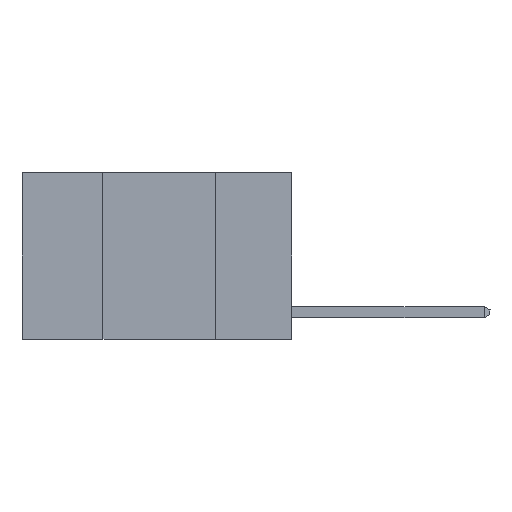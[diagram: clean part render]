
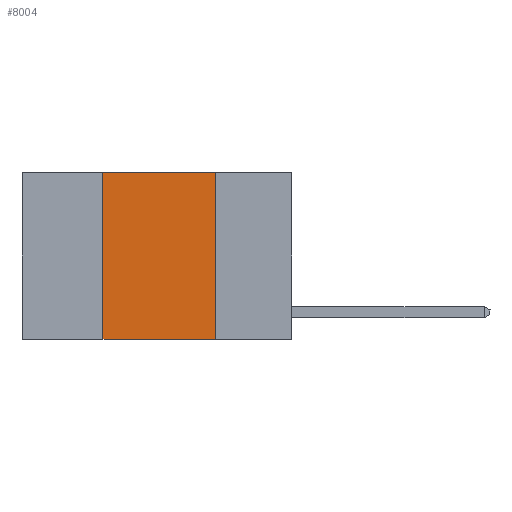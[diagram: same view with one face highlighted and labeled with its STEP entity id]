
A CAD part, left-side view. The second image highlights one B-rep face of the part: STEP entity #8004.
In plain terms, the highlighted planar face has unit normal (-1, 0, 0).
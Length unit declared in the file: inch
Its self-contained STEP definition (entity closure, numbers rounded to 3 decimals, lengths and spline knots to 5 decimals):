
#1813 = VERTEX_POINT ( 'NONE', #27494 ) ;
#3294 = LINE ( 'NONE', #10747, #24729 ) ;
#3376 = AXIS2_PLACEMENT_3D ( 'NONE', #18849, #20961, #8152 ) ;
#3519 = CARTESIAN_POINT ( 'NONE',  ( 0., 0.6, 0. ) ) ;
#3807 = ORIENTED_EDGE ( 'NONE', *, *, #9992, .F. ) ;
#5625 = EDGE_CURVE ( 'NONE', #9618, #1813, #24249, .T. ) ;
#6098 = VECTOR ( 'NONE', #22784, 39.37008 ) ;
#7294 = CARTESIAN_POINT ( 'NONE',  ( 0., 0.17, 0. ) ) ;
#7658 = CARTESIAN_POINT ( 'NONE',  ( 0., 0.42, 0. ) ) ;
#8004 = ADVANCED_FACE ( 'NONE', ( #25153 ), #18753, .F. ) ;
#8152 = DIRECTION ( 'NONE',  ( 0., 0., -1. ) ) ;
#8537 = EDGE_CURVE ( 'NONE', #16854, #9618, #11808, .T. ) ;
#9618 = VERTEX_POINT ( 'NONE', #18137 ) ;
#9623 = EDGE_LOOP ( 'NONE', ( #19580, #25844, #3807, #15947 ) ) ;
#9992 = EDGE_CURVE ( 'NONE', #15444, #16854, #3294, .T. ) ;
#10747 = CARTESIAN_POINT ( 'NONE',  ( 0., 0.42, 0. ) ) ;
#11808 = LINE ( 'NONE', #3519, #6098 ) ;
#12515 = CARTESIAN_POINT ( 'NONE',  ( 0., 0.42, -0.37 ) ) ;
#15436 = DIRECTION ( 'NONE',  ( 0., -1., 0. ) ) ;
#15444 = VERTEX_POINT ( 'NONE', #12515 ) ;
#15947 = ORIENTED_EDGE ( 'NONE', *, *, #21604, .T. ) ;
#16854 = VERTEX_POINT ( 'NONE', #7658 ) ;
#17151 = VECTOR ( 'NONE', #15436, 39.37008 ) ;
#18137 = CARTESIAN_POINT ( 'NONE',  ( 0., 0.17, 0. ) ) ;
#18753 = PLANE ( 'NONE',  #3376 ) ;
#18849 = CARTESIAN_POINT ( 'NONE',  ( 0., 0.6, 0. ) ) ;
#19580 = ORIENTED_EDGE ( 'NONE', *, *, #5625, .F. ) ;
#20961 = DIRECTION ( 'NONE',  ( 1., 0., 0. ) ) ;
#21473 = DIRECTION ( 'NONE',  ( 0., 0., 1. ) ) ;
#21604 = EDGE_CURVE ( 'NONE', #15444, #1813, #22768, .T. ) ;
#21736 = CARTESIAN_POINT ( 'NONE',  ( 0., 0.6, -0.37 ) ) ;
#22237 = DIRECTION ( 'NONE',  ( 0., 0., -1. ) ) ;
#22768 = LINE ( 'NONE', #21736, #17151 ) ;
#22784 = DIRECTION ( 'NONE',  ( 0., -1., 0. ) ) ;
#24249 = LINE ( 'NONE', #7294, #24899 ) ;
#24729 = VECTOR ( 'NONE', #21473, 39.37008 ) ;
#24899 = VECTOR ( 'NONE', #22237, 39.37008 ) ;
#25153 = FACE_OUTER_BOUND ( 'NONE', #9623, .T. ) ;
#25844 = ORIENTED_EDGE ( 'NONE', *, *, #8537, .F. ) ;
#27494 = CARTESIAN_POINT ( 'NONE',  ( 0., 0.17, -0.37 ) ) ;
